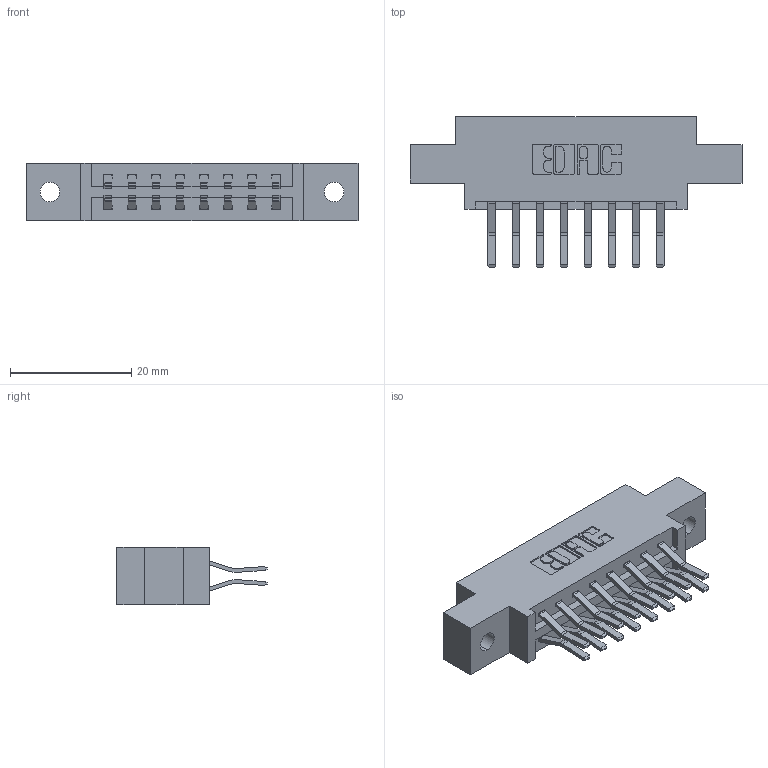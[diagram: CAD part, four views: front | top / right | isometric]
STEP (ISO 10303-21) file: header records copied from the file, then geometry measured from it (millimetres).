
FILE_DESCRIPTION (( 'STEP AP203' ), '1' );
FILE_NAME ('387-016-560-802.STEP', '2019-10-16T00:18:02', ( '' ), ( '' ), 'SwSTEP 2.0', 'SolidWorks 2016', '' );
FILE_SCHEMA (( 'CONFIG_CONTROL_DESIGN' ));
Length unit declared in the file: inch
Products named in the file (3): 387-016-560-802; 345-292-001_560 Tail; 337 Part_0.170 Offset - 0.128 Dia
Assembly tree (17 placements, depth 2):
  387-016-560-802
    337 Part_0.170 Offset - 0.128 Dia
    345-292-001_560 Tail  x16
Bounding box: 54.71 x 24.78 x 9.4 mm (x, y, z)
Volume: 5264.1 mm3; surface area: 5759.4 mm2
Topology: 17 solids, 17 shells, 1014 faces, 2995 edges, 1974 vertices
Faces by surface type: plane 682, cylinder 332
Entity records: 10823 total; most frequent: CARTESIAN_POINT 1854, ORIENTED_EDGE 1790, DIRECTION 1643, EDGE_CURVE 895, VECTOR 763, LINE 763, VERTEX_POINT 594, AXIS2_PLACEMENT_3D 440
